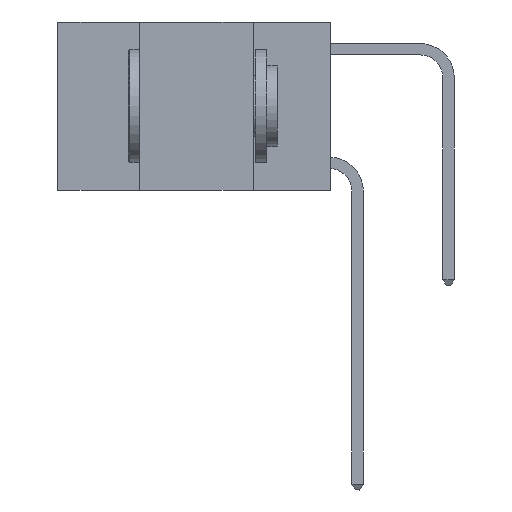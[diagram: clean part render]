
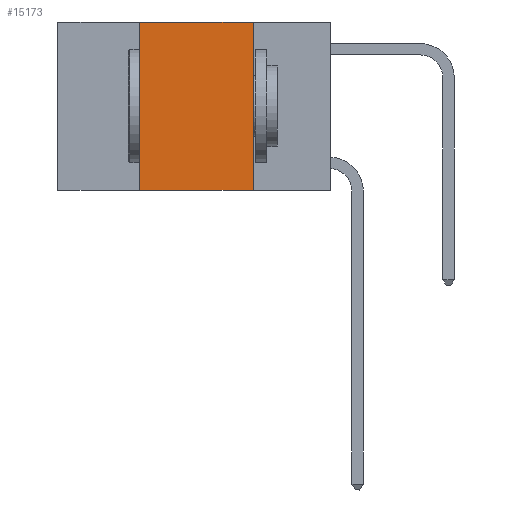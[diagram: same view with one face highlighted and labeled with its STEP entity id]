
A CAD part, left-side view. The second image highlights one B-rep face of the part: STEP entity #15173.
In plain terms, the highlighted planar face has unit normal (-1, 0, 0).
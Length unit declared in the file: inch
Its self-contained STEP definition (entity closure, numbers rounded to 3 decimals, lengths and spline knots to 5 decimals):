
#70 = EDGE_CURVE ( 'NONE', #4613, #1023, #12117, .T. ) ;
#739 = VERTEX_POINT ( 'NONE', #22158 ) ;
#1023 = VERTEX_POINT ( 'NONE', #10572 ) ;
#1220 = DIRECTION ( 'NONE',  ( 0., 0., -1. ) ) ;
#1382 = EDGE_CURVE ( 'NONE', #18775, #1023, #3974, .T. ) ;
#1601 = LINE ( 'NONE', #1740, #15379 ) ;
#1740 = CARTESIAN_POINT ( 'NONE',  ( 0., 0.42, 0. ) ) ;
#3805 = LINE ( 'NONE', #12721, #21263 ) ;
#3974 = LINE ( 'NONE', #16989, #19887 ) ;
#4613 = VERTEX_POINT ( 'NONE', #10330 ) ;
#5266 = DIRECTION ( 'NONE',  ( 0., -1., 0. ) ) ;
#6559 = DIRECTION ( 'NONE',  ( 0., 0., 1. ) ) ;
#7429 = VECTOR ( 'NONE', #5266, 39.37008 ) ;
#7441 = CARTESIAN_POINT ( 'NONE',  ( 0., 0.6, -0.37 ) ) ;
#7767 = ORIENTED_EDGE ( 'NONE', *, *, #28384, .F. ) ;
#7939 = EDGE_LOOP ( 'NONE', ( #9602, #10698, #7767, #20482 ) ) ;
#8618 = DIRECTION ( 'NONE',  ( 0., -1., 0. ) ) ;
#9602 = ORIENTED_EDGE ( 'NONE', *, *, #1382, .F. ) ;
#10067 = CARTESIAN_POINT ( 'NONE',  ( 0., 0.17, 0. ) ) ;
#10157 = FACE_OUTER_BOUND ( 'NONE', #7939, .T. ) ;
#10330 = CARTESIAN_POINT ( 'NONE',  ( 0., 0.42, -0.37 ) ) ;
#10572 = CARTESIAN_POINT ( 'NONE',  ( 0., 0.17, -0.37 ) ) ;
#10698 = ORIENTED_EDGE ( 'NONE', *, *, #14375, .F. ) ;
#12117 = LINE ( 'NONE', #7441, #7429 ) ;
#12227 = PLANE ( 'NONE',  #28294 ) ;
#12721 = CARTESIAN_POINT ( 'NONE',  ( 0., 0.6, 0. ) ) ;
#14276 = DIRECTION ( 'NONE',  ( 0., 0., -1. ) ) ;
#14375 = EDGE_CURVE ( 'NONE', #739, #18775, #3805, .T. ) ;
#15173 = ADVANCED_FACE ( 'NONE', ( #10157 ), #12227, .F. ) ;
#15379 = VECTOR ( 'NONE', #6559, 39.37008 ) ;
#16989 = CARTESIAN_POINT ( 'NONE',  ( 0., 0.17, 0. ) ) ;
#18775 = VERTEX_POINT ( 'NONE', #10067 ) ;
#19887 = VECTOR ( 'NONE', #1220, 39.37008 ) ;
#20482 = ORIENTED_EDGE ( 'NONE', *, *, #70, .T. ) ;
#20990 = DIRECTION ( 'NONE',  ( 1., 0., 0. ) ) ;
#21263 = VECTOR ( 'NONE', #8618, 39.37008 ) ;
#22158 = CARTESIAN_POINT ( 'NONE',  ( 0., 0.42, 0. ) ) ;
#28018 = CARTESIAN_POINT ( 'NONE',  ( 0., 0.6, 0. ) ) ;
#28294 = AXIS2_PLACEMENT_3D ( 'NONE', #28018, #20990, #14276 ) ;
#28384 = EDGE_CURVE ( 'NONE', #4613, #739, #1601, .T. ) ;
